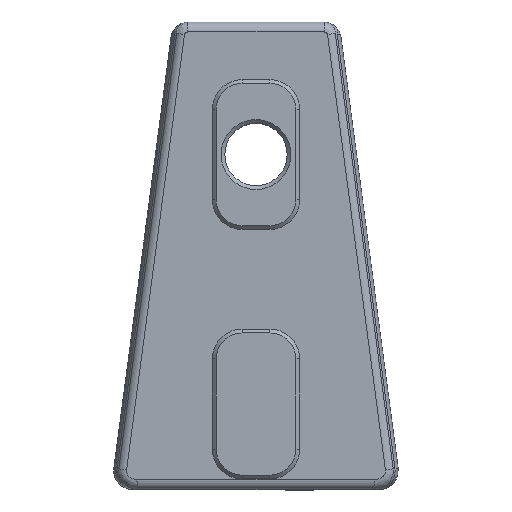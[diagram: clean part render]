
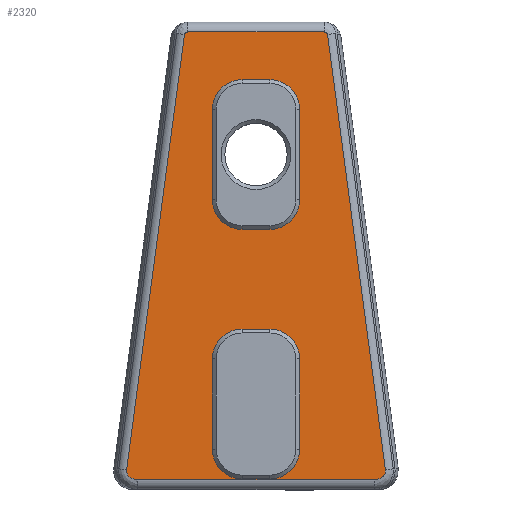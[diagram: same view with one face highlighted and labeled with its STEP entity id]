
A CAD part, top view. The second image highlights one B-rep face of the part: STEP entity #2320.
In plain terms, the highlighted planar face has unit normal (0, 0, 1).
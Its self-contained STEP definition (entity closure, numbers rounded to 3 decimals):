
#26=ELLIPSE('',#2550,0.891,0.7);
#28=ELLIPSE('',#2558,0.891,0.7);
#44=FACE_BOUND('',#743,.T.);
#45=FACE_BOUND('',#744,.T.);
#104=PLANE('',#2566);
#187=LINE('',#4077,#335);
#190=LINE('',#4085,#338);
#210=LINE('',#4143,#358);
#213=LINE('',#4151,#361);
#220=LINE('',#4174,#368);
#221=LINE('',#4176,#369);
#245=LINE('',#5111,#393);
#246=LINE('',#5149,#394);
#247=LINE('',#5155,#395);
#250=LINE('',#5236,#398);
#254=LINE('',#5255,#402);
#255=LINE('',#5256,#403);
#335=VECTOR('',#2902,10.);
#338=VECTOR('',#2911,10.);
#358=VECTOR('',#2969,10.);
#361=VECTOR('',#2978,10.);
#368=VECTOR('',#3005,10.);
#369=VECTOR('',#3008,10.);
#393=VECTOR('',#3104,10.);
#394=VECTOR('',#3115,10.);
#395=VECTOR('',#3120,10.);
#398=VECTOR('',#3133,10.);
#402=VECTOR('',#3151,10.);
#403=VECTOR('',#3152,10.);
#581=FACE_OUTER_BOUND('',#742,.T.);
#742=EDGE_LOOP('',(#2000,#2001,#2002,#2003,#2004,#2005,#2006,#2007));
#743=EDGE_LOOP('',(#2008,#2009,#2010,#2011,#2012,#2013,#2014,#2015));
#744=EDGE_LOOP('',(#2016,#2017,#2018,#2019,#2020,#2021,#2022,#2023));
#817=B_SPLINE_CURVE_WITH_KNOTS('',3,(#5101,#5102,#5103,#5104,#5105),
 .UNSPECIFIED.,.F.,.F.,(4,1,4),(0.,0.015,0.035),
 .UNSPECIFIED.);
#819=B_SPLINE_CURVE_WITH_KNOTS('',3,(#5197,#5198,#5199,#5200,#5201),
 .UNSPECIFIED.,.F.,.F.,(4,1,4),(0.,0.02,
0.035),.UNSPECIFIED.);
#898=CIRCLE('',#2474,2.38);
#899=CIRCLE('',#2477,2.38);
#908=CIRCLE('',#2496,2.38);
#909=CIRCLE('',#2499,2.38);
#910=CIRCLE('',#2503,2.38);
#911=CIRCLE('',#2505,2.38);
#912=CIRCLE('',#2507,2.38);
#913=CIRCLE('',#2509,2.38);
#1038=VERTEX_POINT('',#4069);
#1039=VERTEX_POINT('',#4071);
#1040=VERTEX_POINT('',#4075);
#1041=VERTEX_POINT('',#4079);
#1042=VERTEX_POINT('',#4083);
#1059=VERTEX_POINT('',#4135);
#1060=VERTEX_POINT('',#4137);
#1061=VERTEX_POINT('',#4141);
#1062=VERTEX_POINT('',#4145);
#1063=VERTEX_POINT('',#4149);
#1064=VERTEX_POINT('',#4154);
#1065=VERTEX_POINT('',#4156);
#1066=VERTEX_POINT('',#4160);
#1067=VERTEX_POINT('',#4164);
#1068=VERTEX_POINT('',#4166);
#1069=VERTEX_POINT('',#4170);
#1096=VERTEX_POINT('',#5090);
#1099=VERTEX_POINT('',#5099);
#1100=VERTEX_POINT('',#5107);
#1102=VERTEX_POINT('',#5142);
#1103=VERTEX_POINT('',#5147);
#1105=VERTEX_POINT('',#5152);
#1106=VERTEX_POINT('',#5154);
#1108=VERTEX_POINT('',#5189);
#1289=EDGE_CURVE('',#1039,#1038,#898,.T.);
#1292=EDGE_CURVE('',#1038,#1040,#187,.T.);
#1294=EDGE_CURVE('',#1040,#1041,#899,.T.);
#1296=EDGE_CURVE('',#1041,#1042,#190,.F.);
#1322=EDGE_CURVE('',#1059,#1060,#908,.T.);
#1325=EDGE_CURVE('',#1061,#1059,#210,.T.);
#1327=EDGE_CURVE('',#1062,#1061,#909,.T.);
#1329=EDGE_CURVE('',#1062,#1063,#213,.F.);
#1331=EDGE_CURVE('',#1064,#1065,#910,.T.);
#1334=EDGE_CURVE('',#1066,#1042,#911,.T.);
#1336=EDGE_CURVE('',#1068,#1067,#912,.T.);
#1339=EDGE_CURVE('',#1063,#1069,#913,.T.);
#1340=EDGE_CURVE('',#1065,#1066,#220,.T.);
#1341=EDGE_CURVE('',#1069,#1068,#221,.T.);
#1397=EDGE_CURVE('',#1099,#1096,#817,.T.);
#1400=EDGE_CURVE('',#1096,#1100,#245,.T.);
#1403=EDGE_CURVE('',#1100,#1102,#26,.T.);
#1405=EDGE_CURVE('',#1102,#1103,#246,.T.);
#1407=EDGE_CURVE('',#1105,#1106,#247,.T.);
#1412=EDGE_CURVE('',#1106,#1108,#819,.T.);
#1414=EDGE_CURVE('',#1103,#1105,#28,.T.);
#1416=EDGE_CURVE('',#1108,#1099,#250,.T.);
#1424=EDGE_CURVE('',#1060,#1067,#254,.T.);
#1425=EDGE_CURVE('',#1039,#1064,#255,.T.);
#2000=ORIENTED_EDGE('',*,*,#1407,.F.);
#2001=ORIENTED_EDGE('',*,*,#1414,.F.);
#2002=ORIENTED_EDGE('',*,*,#1405,.F.);
#2003=ORIENTED_EDGE('',*,*,#1403,.F.);
#2004=ORIENTED_EDGE('',*,*,#1400,.F.);
#2005=ORIENTED_EDGE('',*,*,#1397,.F.);
#2006=ORIENTED_EDGE('',*,*,#1416,.F.);
#2007=ORIENTED_EDGE('',*,*,#1412,.F.);
#2008=ORIENTED_EDGE('',*,*,#1329,.T.);
#2009=ORIENTED_EDGE('',*,*,#1339,.T.);
#2010=ORIENTED_EDGE('',*,*,#1341,.T.);
#2011=ORIENTED_EDGE('',*,*,#1336,.T.);
#2012=ORIENTED_EDGE('',*,*,#1424,.F.);
#2013=ORIENTED_EDGE('',*,*,#1322,.F.);
#2014=ORIENTED_EDGE('',*,*,#1325,.F.);
#2015=ORIENTED_EDGE('',*,*,#1327,.F.);
#2016=ORIENTED_EDGE('',*,*,#1334,.F.);
#2017=ORIENTED_EDGE('',*,*,#1340,.F.);
#2018=ORIENTED_EDGE('',*,*,#1331,.F.);
#2019=ORIENTED_EDGE('',*,*,#1425,.F.);
#2020=ORIENTED_EDGE('',*,*,#1289,.T.);
#2021=ORIENTED_EDGE('',*,*,#1292,.T.);
#2022=ORIENTED_EDGE('',*,*,#1294,.T.);
#2023=ORIENTED_EDGE('',*,*,#1296,.T.);
#2320=ADVANCED_FACE('',(#581,#44,#45),#104,.F.);
#2474=AXIS2_PLACEMENT_3D('',#4072,#2896,#2897);
#2477=AXIS2_PLACEMENT_3D('',#4081,#2906,#2907);
#2496=AXIS2_PLACEMENT_3D('',#4138,#2963,#2964);
#2499=AXIS2_PLACEMENT_3D('',#4147,#2973,#2974);
#2503=AXIS2_PLACEMENT_3D('',#4157,#2984,#2985);
#2505=AXIS2_PLACEMENT_3D('',#4162,#2990,#2991);
#2507=AXIS2_PLACEMENT_3D('',#4167,#2995,#2996);
#2509=AXIS2_PLACEMENT_3D('',#4172,#3001,#3002);
#2550=AXIS2_PLACEMENT_3D('',#5145,#3109,#3110);
#2558=AXIS2_PLACEMENT_3D('',#5233,#3128,#3129);
#2566=AXIS2_PLACEMENT_3D('',#5254,#3149,#3150);
#2896=DIRECTION('center_axis',(0.,0.,-1.));
#2897=DIRECTION('ref_axis',(0.,1.,0.));
#2902=DIRECTION('',(1.,0.,0.));
#2906=DIRECTION('center_axis',(0.,0.,-1.));
#2907=DIRECTION('ref_axis',(1.,0.,0.));
#2911=DIRECTION('',(0.,1.,0.));
#2963=DIRECTION('center_axis',(0.,0.,1.));
#2964=DIRECTION('ref_axis',(0.,1.,0.));
#2969=DIRECTION('',(-1.,0.,0.));
#2973=DIRECTION('center_axis',(0.,0.,1.));
#2974=DIRECTION('ref_axis',(1.,0.,0.));
#2978=DIRECTION('',(0.,1.,0.));
#2984=DIRECTION('center_axis',(0.,0.,1.));
#2985=DIRECTION('ref_axis',(-1.,0.,0.));
#2990=DIRECTION('center_axis',(0.,0.,1.));
#2991=DIRECTION('ref_axis',(0.,-1.,0.));
#2995=DIRECTION('center_axis',(0.,0.,-1.));
#2996=DIRECTION('ref_axis',(-1.,0.,0.));
#3001=DIRECTION('center_axis',(0.,0.,-1.));
#3002=DIRECTION('ref_axis',(0.,-1.,0.));
#3005=DIRECTION('',(1.,0.,0.));
#3008=DIRECTION('',(-1.,0.,0.));
#3104=DIRECTION('',(0.132,-0.991,0.));
#3109=DIRECTION('center_axis',(0.,0.,-1.));
#3110=DIRECTION('ref_axis',(1.,0.,0.));
#3115=DIRECTION('',(-1.,0.,0.));
#3120=DIRECTION('',(0.132,0.991,0.));
#3128=DIRECTION('center_axis',(0.,0.,-1.));
#3129=DIRECTION('ref_axis',(-1.,0.,0.));
#3133=DIRECTION('',(1.,0.,0.));
#3149=DIRECTION('center_axis',(0.,0.,-1.));
#3150=DIRECTION('ref_axis',(1.,0.,0.));
#3151=DIRECTION('',(0.,-1.,0.));
#3152=DIRECTION('',(0.,-1.,0.));
#4069=CARTESIAN_POINT('',(-1.12,39.1,-1.));
#4071=CARTESIAN_POINT('',(-3.5,36.72,-1.));
#4072=CARTESIAN_POINT('Origin',(-1.12,36.72,-1.));
#4075=CARTESIAN_POINT('',(1.12,39.1,-1.));
#4077=CARTESIAN_POINT('',(-0.56,39.1,-1.));
#4079=CARTESIAN_POINT('',(3.5,36.72,-1.));
#4081=CARTESIAN_POINT('Origin',(1.12,36.72,-1.));
#4083=CARTESIAN_POINT('',(3.5,29.48,-1.));
#4085=CARTESIAN_POINT('',(3.5,5.35,-1.));
#4135=CARTESIAN_POINT('',(-1.12,19.1,-1.));
#4137=CARTESIAN_POINT('',(-3.5,16.72,-1.));
#4138=CARTESIAN_POINT('Origin',(-1.12,16.72,-1.));
#4141=CARTESIAN_POINT('',(1.12,19.1,-1.));
#4143=CARTESIAN_POINT('',(0.56,19.1,-1.));
#4145=CARTESIAN_POINT('',(3.5,16.72,-1.));
#4147=CARTESIAN_POINT('Origin',(1.12,16.72,-1.));
#4149=CARTESIAN_POINT('',(3.5,9.48,-1.));
#4151=CARTESIAN_POINT('',(3.5,5.35,-1.));
#4154=CARTESIAN_POINT('',(-3.5,29.48,-1.));
#4156=CARTESIAN_POINT('',(-1.12,27.1,-1.));
#4157=CARTESIAN_POINT('Origin',(-1.12,29.48,-1.));
#4160=CARTESIAN_POINT('',(1.12,27.1,-1.));
#4162=CARTESIAN_POINT('Origin',(1.12,29.48,-1.));
#4164=CARTESIAN_POINT('',(-3.5,9.48,-1.));
#4166=CARTESIAN_POINT('',(-1.12,7.1,-1.));
#4167=CARTESIAN_POINT('Origin',(-1.12,9.48,-1.));
#4170=CARTESIAN_POINT('',(1.12,7.1,-1.));
#4172=CARTESIAN_POINT('Origin',(1.12,9.48,-1.));
#4174=CARTESIAN_POINT('',(-0.56,27.1,-1.));
#4176=CARTESIAN_POINT('',(0.56,7.1,-1.));
#5090=CARTESIAN_POINT('',(5.733,42.73,-1.));
#5099=CARTESIAN_POINT('',(5.473,42.928,-1.));
#5101=CARTESIAN_POINT('Ctrl Pts',(5.473,42.928,-1.));
#5102=CARTESIAN_POINT('Ctrl Pts',(5.524,42.928,-1.));
#5103=CARTESIAN_POINT('Ctrl Pts',(5.64,42.896,-1.));
#5104=CARTESIAN_POINT('Ctrl Pts',(5.724,42.797,-1.));
#5105=CARTESIAN_POINT('Ctrl Pts',(5.733,42.73,-1.));
#5107=CARTESIAN_POINT('',(10.371,7.823,-1.));
#5111=CARTESIAN_POINT('',(7.54,29.131,-1.));
#5142=CARTESIAN_POINT('',(9.485,7.05,-1.));
#5145=CARTESIAN_POINT('Origin',(9.485,7.75,-1.));
#5147=CARTESIAN_POINT('',(-9.485,7.05,-1.));
#5149=CARTESIAN_POINT('',(0.56,7.05,-1.));
#5152=CARTESIAN_POINT('',(-10.371,7.823,-1.));
#5154=CARTESIAN_POINT('',(-5.733,42.73,-1.));
#5155=CARTESIAN_POINT('',(-8.719,20.256,-1.));
#5189=CARTESIAN_POINT('',(-5.473,42.928,-1.));
#5197=CARTESIAN_POINT('Ctrl Pts',(-5.733,42.73,-1.));
#5198=CARTESIAN_POINT('Ctrl Pts',(-5.724,42.797,-1.));
#5199=CARTESIAN_POINT('Ctrl Pts',(-5.64,42.896,-1.));
#5200=CARTESIAN_POINT('Ctrl Pts',(-5.524,42.928,-1.));
#5201=CARTESIAN_POINT('Ctrl Pts',(-5.473,42.928,-1.));
#5233=CARTESIAN_POINT('Origin',(-9.485,7.75,-1.));
#5236=CARTESIAN_POINT('',(0.,42.928,-1.));
#5254=CARTESIAN_POINT('Origin',(0.,24.,-1.));
#5255=CARTESIAN_POINT('',(-3.5,5.35,-1.));
#5256=CARTESIAN_POINT('',(-3.5,5.35,-1.));
